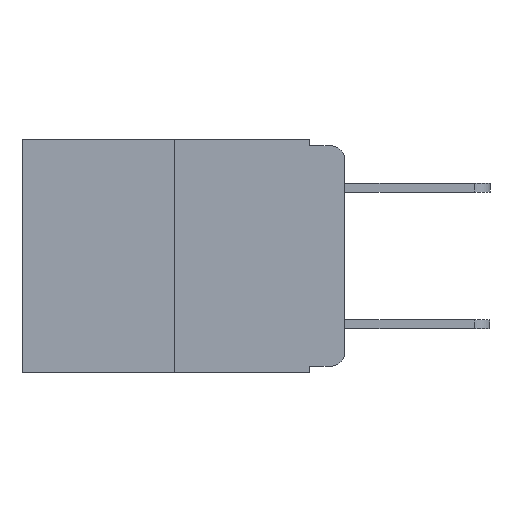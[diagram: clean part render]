
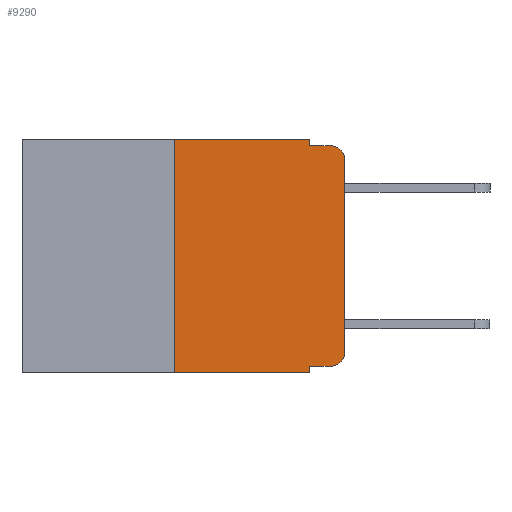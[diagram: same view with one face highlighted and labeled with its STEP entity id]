
A CAD part, left-side view. The second image highlights one B-rep face of the part: STEP entity #9290.
In plain terms, the highlighted planar face has unit normal (-1, 0, 0).
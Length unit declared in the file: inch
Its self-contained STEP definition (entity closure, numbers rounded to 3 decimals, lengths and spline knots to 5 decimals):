
#98 = PLANE ( 'NONE',  #17270 ) ;
#137 = DIRECTION ( 'NONE',  ( -1., 0., 0. ) ) ;
#229 = CARTESIAN_POINT ( 'NONE',  ( 0., 0.473, -0.343 ) ) ;
#276 = EDGE_CURVE ( 'NONE', #8898, #2627, #19157, .T. ) ;
#526 = CARTESIAN_POINT ( 'NONE',  ( 0., 0.051, -0.333 ) ) ;
#1391 = VECTOR ( 'NONE', #18336, 39.37008 ) ;
#1642 = CARTESIAN_POINT ( 'NONE',  ( 0., 0.051, -0.333 ) ) ;
#1991 = LINE ( 'NONE', #1642, #1391 ) ;
#2060 = DIRECTION ( 'NONE',  ( 1., 0., 0. ) ) ;
#2150 = CARTESIAN_POINT ( 'NONE',  ( 0., 0.051, -0.01 ) ) ;
#2214 = CARTESIAN_POINT ( 'NONE',  ( 0., 0.02, -0.01 ) ) ;
#2627 = VERTEX_POINT ( 'NONE', #16990 ) ;
#3307 = VERTEX_POINT ( 'NONE', #11404 ) ;
#3467 = VERTEX_POINT ( 'NONE', #526 ) ;
#3620 = ORIENTED_EDGE ( 'NONE', *, *, #7968, .T. ) ;
#3980 = CIRCLE ( 'NONE', #21331, 0.02 ) ;
#4091 = DIRECTION ( 'NONE',  ( 0., 0., -1. ) ) ;
#4298 = DIRECTION ( 'NONE',  ( 0., -1., 0. ) ) ;
#4776 = VERTEX_POINT ( 'NONE', #2214 ) ;
#5228 = VECTOR ( 'NONE', #18525, 39.37008 ) ;
#5948 = CARTESIAN_POINT ( 'NONE',  ( 0., 0.051, 0. ) ) ;
#6018 = EDGE_CURVE ( 'NONE', #3307, #7486, #8312, .T. ) ;
#6079 = VECTOR ( 'NONE', #22284, 39.37008 ) ;
#6091 = VERTEX_POINT ( 'NONE', #19270 ) ;
#7486 = VERTEX_POINT ( 'NONE', #22213 ) ;
#7710 = VERTEX_POINT ( 'NONE', #14165 ) ;
#7968 = EDGE_CURVE ( 'NONE', #7486, #6091, #18687, .T. ) ;
#8312 = CIRCLE ( 'NONE', #23229, 0.02 ) ;
#8898 = VERTEX_POINT ( 'NONE', #13968 ) ;
#9153 = EDGE_CURVE ( 'NONE', #3467, #3307, #1991, .T. ) ;
#9198 = LINE ( 'NONE', #229, #17686 ) ;
#9290 = ADVANCED_FACE ( 'NONE', ( #18284 ), #98, .F. ) ;
#9332 = EDGE_CURVE ( 'NONE', #2627, #4776, #17701, .T. ) ;
#9434 = DIRECTION ( 'NONE',  ( 0., 0., 1. ) ) ;
#9489 = CARTESIAN_POINT ( 'NONE',  ( 0., 0.25, 0. ) ) ;
#9849 = DIRECTION ( 'NONE',  ( 0., -1., 0. ) ) ;
#9915 = EDGE_CURVE ( 'NONE', #12450, #8898, #15380, .T. ) ;
#10019 = CARTESIAN_POINT ( 'NONE',  ( 0., 0.02, -0.313 ) ) ;
#10146 = ORIENTED_EDGE ( 'NONE', *, *, #9915, .F. ) ;
#10474 = CARTESIAN_POINT ( 'NONE',  ( 0., 0.051, 0. ) ) ;
#10954 = LINE ( 'NONE', #5948, #6079 ) ;
#11404 = CARTESIAN_POINT ( 'NONE',  ( 0., 0.02, -0.333 ) ) ;
#11542 = CARTESIAN_POINT ( 'NONE',  ( 0., 0.02, -0.03 ) ) ;
#11846 = DIRECTION ( 'NONE',  ( 0., 0., -1. ) ) ;
#12161 = ORIENTED_EDGE ( 'NONE', *, *, #9153, .T. ) ;
#12450 = VERTEX_POINT ( 'NONE', #15088 ) ;
#12870 = VECTOR ( 'NONE', #9849, 39.37008 ) ;
#13052 = CARTESIAN_POINT ( 'NONE',  ( 0., 0., 0. ) ) ;
#13317 = CARTESIAN_POINT ( 'NONE',  ( 0., 0.473, 0. ) ) ;
#13343 = DIRECTION ( 'NONE',  ( 0., 0., -1. ) ) ;
#13813 = ORIENTED_EDGE ( 'NONE', *, *, #276, .F. ) ;
#13968 = CARTESIAN_POINT ( 'NONE',  ( 0., 0.051, 0. ) ) ;
#14165 = CARTESIAN_POINT ( 'NONE',  ( 0., 0.051, -0.343 ) ) ;
#14240 = VECTOR ( 'NONE', #21761, 39.37008 ) ;
#14667 = ORIENTED_EDGE ( 'NONE', *, *, #21259, .F. ) ;
#14957 = LINE ( 'NONE', #9489, #5228 ) ;
#15088 = CARTESIAN_POINT ( 'NONE',  ( 0., 0.25, 0. ) ) ;
#15120 = DIRECTION ( 'NONE',  ( 0., 0., -1. ) ) ;
#15380 = LINE ( 'NONE', #18249, #14240 ) ;
#15495 = ORIENTED_EDGE ( 'NONE', *, *, #19165, .F. ) ;
#15766 = ORIENTED_EDGE ( 'NONE', *, *, #19235, .T. ) ;
#16087 = EDGE_CURVE ( 'NONE', #22199, #7710, #9198, .T. ) ;
#16990 = CARTESIAN_POINT ( 'NONE',  ( 0., 0.051, -0.01 ) ) ;
#17270 = AXIS2_PLACEMENT_3D ( 'NONE', #13317, #2060, #15120 ) ;
#17560 = ORIENTED_EDGE ( 'NONE', *, *, #6018, .T. ) ;
#17686 = VECTOR ( 'NONE', #4298, 39.37008 ) ;
#17701 = LINE ( 'NONE', #2150, #12870 ) ;
#18249 = CARTESIAN_POINT ( 'NONE',  ( 0., 0.473, 0. ) ) ;
#18284 = FACE_OUTER_BOUND ( 'NONE', #18507, .T. ) ;
#18336 = DIRECTION ( 'NONE',  ( 0., -1., 0. ) ) ;
#18507 = EDGE_LOOP ( 'NONE', ( #3620, #15766, #21704, #13813, #10146, #15495, #21185, #14667, #12161, #17560 ) ) ;
#18525 = DIRECTION ( 'NONE',  ( 0., 0., 1. ) ) ;
#18599 = VECTOR ( 'NONE', #4091, 39.37008 ) ;
#18687 = LINE ( 'NONE', #13052, #22862 ) ;
#19157 = LINE ( 'NONE', #10474, #18599 ) ;
#19165 = EDGE_CURVE ( 'NONE', #22199, #12450, #14957, .T. ) ;
#19235 = EDGE_CURVE ( 'NONE', #6091, #4776, #3980, .T. ) ;
#19270 = CARTESIAN_POINT ( 'NONE',  ( 0., 0., -0.03 ) ) ;
#19693 = CARTESIAN_POINT ( 'NONE',  ( 0., 0.25, -0.343 ) ) ;
#21185 = ORIENTED_EDGE ( 'NONE', *, *, #16087, .T. ) ;
#21259 = EDGE_CURVE ( 'NONE', #3467, #7710, #10954, .T. ) ;
#21331 = AXIS2_PLACEMENT_3D ( 'NONE', #11542, #137, #13343 ) ;
#21704 = ORIENTED_EDGE ( 'NONE', *, *, #9332, .F. ) ;
#21761 = DIRECTION ( 'NONE',  ( 0., -1., 0. ) ) ;
#22199 = VERTEX_POINT ( 'NONE', #19693 ) ;
#22213 = CARTESIAN_POINT ( 'NONE',  ( 0., 0., -0.313 ) ) ;
#22284 = DIRECTION ( 'NONE',  ( 0., 0., -1. ) ) ;
#22613 = DIRECTION ( 'NONE',  ( -1., 0., 0. ) ) ;
#22862 = VECTOR ( 'NONE', #9434, 39.37008 ) ;
#23229 = AXIS2_PLACEMENT_3D ( 'NONE', #10019, #22613, #11846 ) ;
